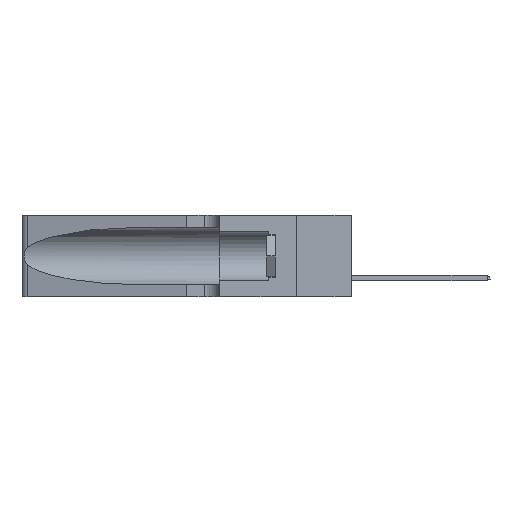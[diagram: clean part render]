
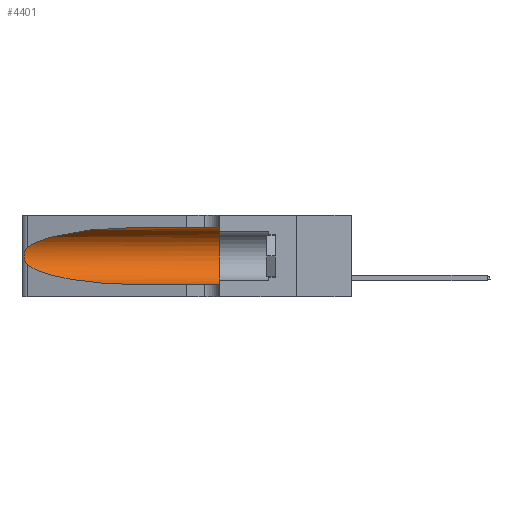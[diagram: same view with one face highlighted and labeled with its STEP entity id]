
A CAD part, left-side view. The second image highlights one B-rep face of the part: STEP entity #4401.
In plain terms, the highlighted cylindrical face has radius 3.308 mm (diameter 6.617 mm), a partial arc.
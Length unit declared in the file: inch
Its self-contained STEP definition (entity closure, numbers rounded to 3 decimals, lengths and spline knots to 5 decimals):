
#608 = CARTESIAN_POINT ( 'NONE',  ( 0.25639, 1.23184, 0.21858 ) ) ;
#1683 = LINE ( 'NONE', #36704, #12834 ) ;
#2875 = AXIS2_PLACEMENT_3D ( 'NONE', #22679, #12962, #39178 ) ;
#3056 = EDGE_LOOP ( 'NONE', ( #6618, #26252, #6795, #22719, #12097, #30236 ) ) ;
#3554 = CYLINDRICAL_SURFACE ( 'NONE', #11869, 0.13025 ) ;
#3593 = CARTESIAN_POINT ( 'NONE',  ( 0.25555, 1.22994, 0.2215 ) ) ;
#3730 = CARTESIAN_POINT ( 'NONE',  ( 0.26018, 1.23835, 0.19895 ) ) ;
#3762 = CARTESIAN_POINT ( 'NONE',  ( 0.1305, 0.72297, 0.31525 ) ) ;
#4148 = CARTESIAN_POINT ( 'NONE',  ( 0.26017, 1.23833, 0.17102 ) ) ;
#4401 = ADVANCED_FACE ( 'NONE', ( #16276 ), #3554, .F. ) ;
#4532 = VERTEX_POINT ( 'NONE', #22189 ) ;
#5155 = VECTOR ( 'NONE', #5937, 39.37008 ) ;
#5937 = DIRECTION ( 'NONE',  ( 0., -1., 0. ) ) ;
#5981 =( BOUNDED_CURVE ( )  B_SPLINE_CURVE ( 3, ( #8639, #8913, #12319, #15536 ),
 .UNSPECIFIED., .F., .F. ) 
 B_SPLINE_CURVE_WITH_KNOTS ( ( 4, 4 ),
 ( 3.44316, 4.71239 ),
 .UNSPECIFIED. ) 
 CURVE ( )  GEOMETRIC_REPRESENTATION_ITEM ( )  RATIONAL_B_SPLINE_CURVE ( ( 1., 0.87, 0.87, 1. ) ) 
 REPRESENTATION_ITEM ( '' )  );
#5987 = CARTESIAN_POINT ( 'NONE',  ( 0.1305, 1.61858, 0.185 ) ) ;
#6502 = CARTESIAN_POINT ( 'NONE',  ( 0.25487, 1.22718, 0.22369 ) ) ;
#6618 = ORIENTED_EDGE ( 'NONE', *, *, #21302, .T. ) ;
#6795 = ORIENTED_EDGE ( 'NONE', *, *, #16702, .T. ) ;
#8639 = CARTESIAN_POINT ( 'NONE',  ( 0.25487, 1.22718, 0.14631 ) ) ;
#8913 = CARTESIAN_POINT ( 'NONE',  ( 0.2373, 1.15595, 0.08982 ) ) ;
#10490 =( BOUNDED_CURVE ( )  B_SPLINE_CURVE ( 3, ( #3762, #29534, #32496, #6502 ),
 .UNSPECIFIED., .F., .F. ) 
 B_SPLINE_CURVE_WITH_KNOTS ( ( 4, 4 ),
 ( 1.5708, 2.84003 ),
 .UNSPECIFIED. ) 
 CURVE ( )  GEOMETRIC_REPRESENTATION_ITEM ( )  RATIONAL_B_SPLINE_CURVE ( ( 1., 0.87, 0.87, 1. ) ) 
 REPRESENTATION_ITEM ( '' )  );
#10744 = CARTESIAN_POINT ( 'NONE',  ( 0.25856, 1.23593, 0.16098 ) ) ;
#11869 = AXIS2_PLACEMENT_3D ( 'NONE', #5987, #25897, #38594 ) ;
#12097 = ORIENTED_EDGE ( 'NONE', *, *, #26184, .F. ) ;
#12243 = B_SPLINE_CURVE_WITH_KNOTS ( 'NONE', 3,
 ( #19923, #3593, #608, #23128, #32473, #3730, #26374, #29652, #4148, #10744, #36255, #29929, #36817, #33307 ),
 .UNSPECIFIED., .F., .F.,
 ( 4, 2, 2, 2, 2, 2, 4 ),
 ( 0., 0.00027, 0.00053, 0.00107, 0.0016, 0.00187, 0.00214 ),
 .UNSPECIFIED. ) ;
#12319 = CARTESIAN_POINT ( 'NONE',  ( 0.18966, 0.96281, 0.05475 ) ) ;
#12834 = VECTOR ( 'NONE', #26688, 39.37008 ) ;
#12962 = DIRECTION ( 'NONE',  ( 0., 1., 0. ) ) ;
#15536 = CARTESIAN_POINT ( 'NONE',  ( 0.1305, 0.72297, 0.05475 ) ) ;
#16276 = FACE_OUTER_BOUND ( 'NONE', #3056, .T. ) ;
#16702 = EDGE_CURVE ( 'NONE', #4532, #17858, #5981, .T. ) ;
#17858 = VERTEX_POINT ( 'NONE', #29334 ) ;
#18254 = CARTESIAN_POINT ( 'NONE',  ( 0.1305, 0.35, 0.31525 ) ) ;
#19923 = CARTESIAN_POINT ( 'NONE',  ( 0.25487, 1.22718, 0.22369 ) ) ;
#21302 = EDGE_CURVE ( 'NONE', #30800, #29353, #10490, .T. ) ;
#21621 = EDGE_CURVE ( 'NONE', #30800, #22787, #24360, .T. ) ;
#22189 = CARTESIAN_POINT ( 'NONE',  ( 0.25487, 1.22718, 0.14631 ) ) ;
#22679 = CARTESIAN_POINT ( 'NONE',  ( 0.1305, 0.35, 0.185 ) ) ;
#22719 = ORIENTED_EDGE ( 'NONE', *, *, #31061, .T. ) ;
#22787 = VERTEX_POINT ( 'NONE', #18254 ) ;
#23128 = CARTESIAN_POINT ( 'NONE',  ( 0.25787, 1.23484, 0.2124 ) ) ;
#24341 = VERTEX_POINT ( 'NONE', #40449 ) ;
#24360 = LINE ( 'NONE', #25147, #5155 ) ;
#25147 = CARTESIAN_POINT ( 'NONE',  ( 0.1305, 1.61858, 0.31525 ) ) ;
#25897 = DIRECTION ( 'NONE',  ( 0., -1., 0. ) ) ;
#26184 = EDGE_CURVE ( 'NONE', #22787, #24341, #33520, .T. ) ;
#26252 = ORIENTED_EDGE ( 'NONE', *, *, #37937, .T. ) ;
#26374 = CARTESIAN_POINT ( 'NONE',  ( 0.26075, 1.23896, 0.19203 ) ) ;
#26688 = DIRECTION ( 'NONE',  ( 0., -1., 0. ) ) ;
#29334 = CARTESIAN_POINT ( 'NONE',  ( 0.1305, 0.72297, 0.05475 ) ) ;
#29353 = VERTEX_POINT ( 'NONE', #41655 ) ;
#29534 = CARTESIAN_POINT ( 'NONE',  ( 0.18966, 0.96281, 0.31525 ) ) ;
#29652 = CARTESIAN_POINT ( 'NONE',  ( 0.26075, 1.23896, 0.178 ) ) ;
#29929 = CARTESIAN_POINT ( 'NONE',  ( 0.25639, 1.23186, 0.15144 ) ) ;
#30236 = ORIENTED_EDGE ( 'NONE', *, *, #21621, .F. ) ;
#30800 = VERTEX_POINT ( 'NONE', #35324 ) ;
#31061 = EDGE_CURVE ( 'NONE', #17858, #24341, #1683, .T. ) ;
#32473 = CARTESIAN_POINT ( 'NONE',  ( 0.25854, 1.2359, 0.20912 ) ) ;
#32496 = CARTESIAN_POINT ( 'NONE',  ( 0.2373, 1.15595, 0.28018 ) ) ;
#33307 = CARTESIAN_POINT ( 'NONE',  ( 0.25487, 1.22718, 0.14631 ) ) ;
#33520 = CIRCLE ( 'NONE', #2875, 0.13025 ) ;
#35324 = CARTESIAN_POINT ( 'NONE',  ( 0.1305, 0.72297, 0.31525 ) ) ;
#36255 = CARTESIAN_POINT ( 'NONE',  ( 0.25789, 1.23486, 0.15765 ) ) ;
#36704 = CARTESIAN_POINT ( 'NONE',  ( 0.1305, 1.61858, 0.05475 ) ) ;
#36817 = CARTESIAN_POINT ( 'NONE',  ( 0.25555, 1.22993, 0.14849 ) ) ;
#37937 = EDGE_CURVE ( 'NONE', #29353, #4532, #12243, .T. ) ;
#38594 = DIRECTION ( 'NONE',  ( 0., 0., -1. ) ) ;
#39178 = DIRECTION ( 'NONE',  ( 0., 0., 1. ) ) ;
#40449 = CARTESIAN_POINT ( 'NONE',  ( 0.1305, 0.35, 0.05475 ) ) ;
#41655 = CARTESIAN_POINT ( 'NONE',  ( 0.25487, 1.22718, 0.22369 ) ) ;
